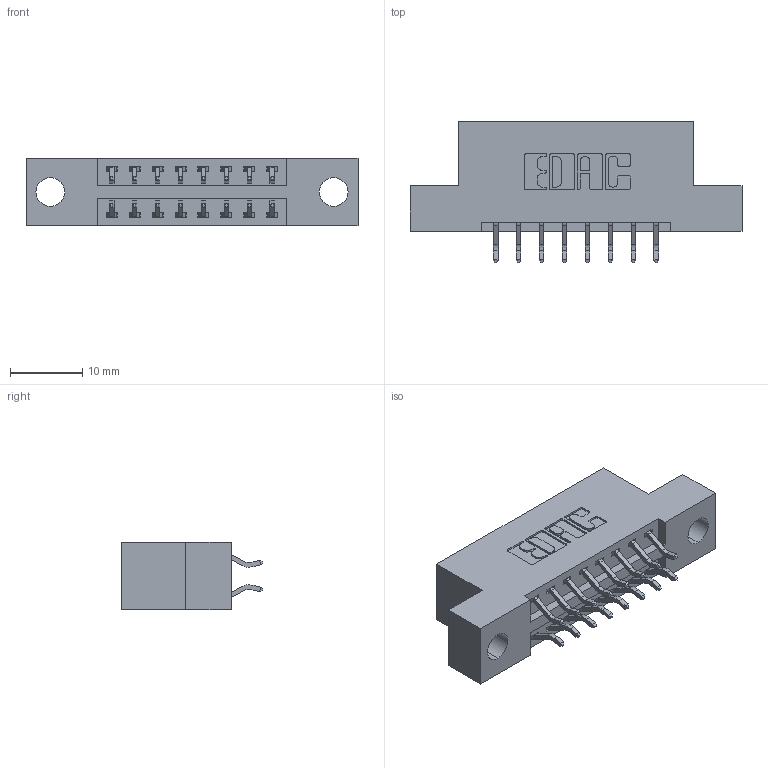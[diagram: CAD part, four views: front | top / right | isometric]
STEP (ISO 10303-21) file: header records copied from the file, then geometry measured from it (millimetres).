
FILE_DESCRIPTION (( 'STEP AP203' ), '1' );
FILE_NAME ('346-016-556-204.STEP', '2022-05-18T16:14:15', ( '' ), ( '' ), 'SwSTEP 2.0', 'SolidWorks 2020', '' );
FILE_SCHEMA (( 'CONFIG_CONTROL_DESIGN' ));
Length unit declared in the file: inch
Products named in the file (3): 346 Part_Flush Mounting Lugs - 0.156 Dia-TH; 345-292-001_556 Tail; 346-016-556-204
Assembly tree (17 placements, depth 2):
  346-016-556-204
    346 Part_Flush Mounting Lugs - 0.156 Dia-TH
    345-292-001_556 Tail  x16
Bounding box: 45.97 x 19.57 x 9.4 mm (x, y, z)
Volume: 4112.4 mm3; surface area: 4951.4 mm2
Topology: 17 solids, 17 shells, 1064 faces, 3133 edges, 2066 vertices
Faces by surface type: plane 714, cylinder 350
Entity records: 10437 total; most frequent: CARTESIAN_POINT 1786, ORIENTED_EDGE 1706, DIRECTION 1613, EDGE_CURVE 853, VECTOR 681, LINE 681, VERTEX_POINT 566, AXIS2_PLACEMENT_3D 466
